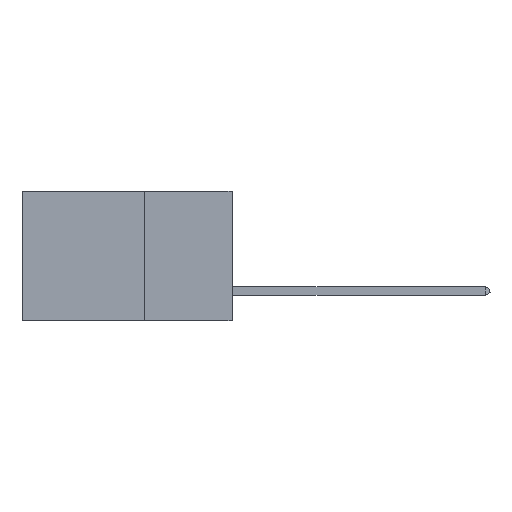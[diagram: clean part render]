
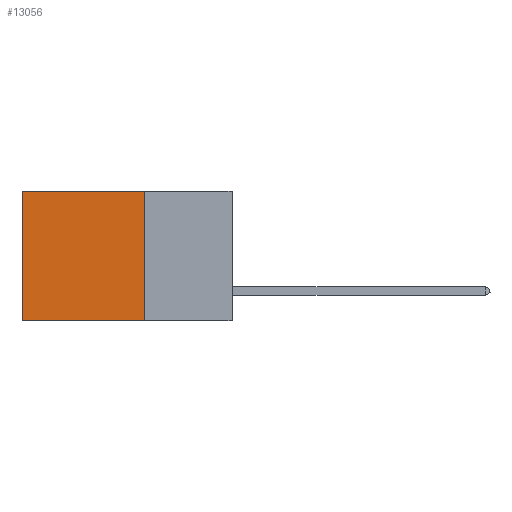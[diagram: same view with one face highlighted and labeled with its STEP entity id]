
A CAD part, left-side view. The second image highlights one B-rep face of the part: STEP entity #13056.
In plain terms, the highlighted planar face has unit normal (-1, 0, 0).
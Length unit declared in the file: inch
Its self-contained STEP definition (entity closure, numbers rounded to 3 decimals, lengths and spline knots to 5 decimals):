
#1428 = DIRECTION ( 'NONE',  ( 0., 0., -1. ) ) ;
#3411 = LINE ( 'NONE', #8458, #32097 ) ;
#3893 = EDGE_CURVE ( 'NONE', #14002, #31842, #18964, .T. ) ;
#5953 = EDGE_CURVE ( 'NONE', #14002, #30397, #3411, .T. ) ;
#6638 = DIRECTION ( 'NONE',  ( 0., 0., -1. ) ) ;
#8458 = CARTESIAN_POINT ( 'NONE',  ( 0.2875, 0.25, 0. ) ) ;
#9002 = LINE ( 'NONE', #16921, #17851 ) ;
#9808 = AXIS2_PLACEMENT_3D ( 'NONE', #22792, #20593, #9823 ) ;
#9823 = DIRECTION ( 'NONE',  ( 0., 0., -1. ) ) ;
#9827 = LINE ( 'NONE', #14714, #10404 ) ;
#10404 = VECTOR ( 'NONE', #20103, 39.37008 ) ;
#11302 = EDGE_CURVE ( 'NONE', #30397, #24228, #9002, .T. ) ;
#13056 = ADVANCED_FACE ( 'NONE', ( #28515 ), #20436, .F. ) ;
#13426 = CARTESIAN_POINT ( 'NONE',  ( 0.2875, 0.25, 0. ) ) ;
#14002 = VERTEX_POINT ( 'NONE', #13426 ) ;
#14660 = EDGE_CURVE ( 'NONE', #31842, #24228, #9827, .T. ) ;
#14714 = CARTESIAN_POINT ( 'NONE',  ( 0.2875, 0.25, -0.37 ) ) ;
#16767 = CARTESIAN_POINT ( 'NONE',  ( 0.2875, 0.25, 0. ) ) ;
#16921 = CARTESIAN_POINT ( 'NONE',  ( 0.2875, 0.6, 0. ) ) ;
#16991 = CARTESIAN_POINT ( 'NONE',  ( 0.2875, 0.6, -0.37 ) ) ;
#17111 = ORIENTED_EDGE ( 'NONE', *, *, #11302, .T. ) ;
#17851 = VECTOR ( 'NONE', #6638, 39.37008 ) ;
#18964 = LINE ( 'NONE', #16767, #19189 ) ;
#19189 = VECTOR ( 'NONE', #1428, 39.37008 ) ;
#19978 = CARTESIAN_POINT ( 'NONE',  ( 0.2875, 0.6, 0. ) ) ;
#20103 = DIRECTION ( 'NONE',  ( 0., 1., 0. ) ) ;
#20436 = PLANE ( 'NONE',  #9808 ) ;
#20593 = DIRECTION ( 'NONE',  ( 1., 0., 0. ) ) ;
#21437 = DIRECTION ( 'NONE',  ( 0., 1., 0. ) ) ;
#22792 = CARTESIAN_POINT ( 'NONE',  ( 0.2875, 0.25, 0. ) ) ;
#23037 = ORIENTED_EDGE ( 'NONE', *, *, #3893, .F. ) ;
#24228 = VERTEX_POINT ( 'NONE', #16991 ) ;
#25018 = ORIENTED_EDGE ( 'NONE', *, *, #14660, .F. ) ;
#26052 = EDGE_LOOP ( 'NONE', ( #17111, #25018, #23037, #31690 ) ) ;
#28515 = FACE_OUTER_BOUND ( 'NONE', #26052, .T. ) ;
#28721 = CARTESIAN_POINT ( 'NONE',  ( 0.2875, 0.25, -0.37 ) ) ;
#30397 = VERTEX_POINT ( 'NONE', #19978 ) ;
#31690 = ORIENTED_EDGE ( 'NONE', *, *, #5953, .T. ) ;
#31842 = VERTEX_POINT ( 'NONE', #28721 ) ;
#32097 = VECTOR ( 'NONE', #21437, 39.37008 ) ;
